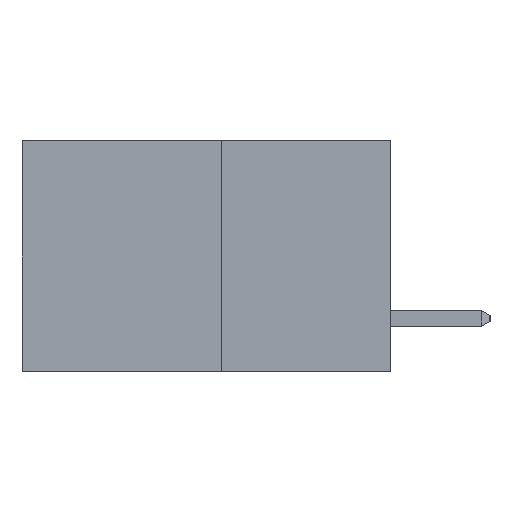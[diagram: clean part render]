
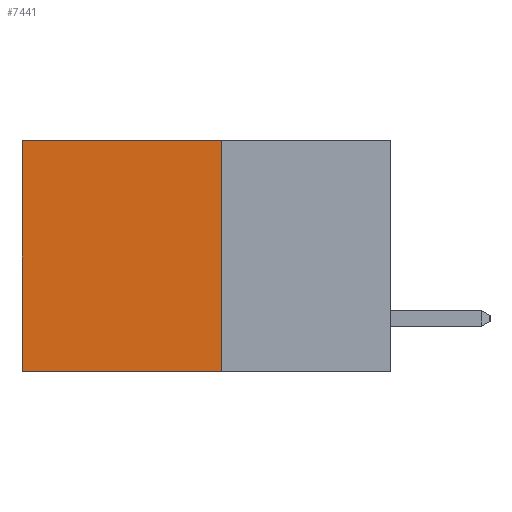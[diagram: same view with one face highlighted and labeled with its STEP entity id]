
A CAD part, left-side view. The second image highlights one B-rep face of the part: STEP entity #7441.
In plain terms, the highlighted planar face has unit normal (-1, 0, 0).
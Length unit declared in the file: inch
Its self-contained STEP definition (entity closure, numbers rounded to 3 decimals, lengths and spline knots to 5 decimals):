
#390 = CARTESIAN_POINT ( 'NONE',  ( 0.277, 0.27, -0.37 ) ) ;
#994 = ORIENTED_EDGE ( 'NONE', *, *, #7520, .T. ) ;
#1193 = CARTESIAN_POINT ( 'NONE',  ( 0.277, 0.27, -0.37 ) ) ;
#1425 = VERTEX_POINT ( 'NONE', #12397 ) ;
#1531 = DIRECTION ( 'NONE',  ( 0., 0., -1. ) ) ;
#1620 = LINE ( 'NONE', #11515, #12965 ) ;
#2081 = AXIS2_PLACEMENT_3D ( 'NONE', #390, #8205, #1531 ) ;
#2526 = CARTESIAN_POINT ( 'NONE',  ( 0.277, 0.27, 0. ) ) ;
#2541 = CARTESIAN_POINT ( 'NONE',  ( 0.277, 0.27, 0. ) ) ;
#3021 = VERTEX_POINT ( 'NONE', #4196 ) ;
#3161 = EDGE_LOOP ( 'NONE', ( #994, #9146, #4348, #8021 ) ) ;
#3484 = LINE ( 'NONE', #1193, #9038 ) ;
#3695 = LINE ( 'NONE', #11509, #6670 ) ;
#3814 = DIRECTION ( 'NONE',  ( 0., 0., -1. ) ) ;
#4196 = CARTESIAN_POINT ( 'NONE',  ( 0.277, 0.59, 0. ) ) ;
#4348 = ORIENTED_EDGE ( 'NONE', *, *, #13926, .F. ) ;
#6143 = LINE ( 'NONE', #2526, #10631 ) ;
#6670 = VECTOR ( 'NONE', #3814, 39.37008 ) ;
#6728 = VERTEX_POINT ( 'NONE', #13368 ) ;
#7095 = PLANE ( 'NONE',  #2081 ) ;
#7197 = DIRECTION ( 'NONE',  ( 0., 0., -1. ) ) ;
#7392 = EDGE_CURVE ( 'NONE', #8718, #3021, #6143, .T. ) ;
#7441 = ADVANCED_FACE ( 'NONE', ( #13134 ), #7095, .F. ) ;
#7520 = EDGE_CURVE ( 'NONE', #3021, #1425, #3695, .T. ) ;
#8021 = ORIENTED_EDGE ( 'NONE', *, *, #7392, .T. ) ;
#8205 = DIRECTION ( 'NONE',  ( 1., 0., 0. ) ) ;
#8608 = EDGE_CURVE ( 'NONE', #6728, #1425, #3484, .T. ) ;
#8718 = VERTEX_POINT ( 'NONE', #2541 ) ;
#9038 = VECTOR ( 'NONE', #11174, 39.37008 ) ;
#9146 = ORIENTED_EDGE ( 'NONE', *, *, #8608, .F. ) ;
#10631 = VECTOR ( 'NONE', #11392, 39.37008 ) ;
#11174 = DIRECTION ( 'NONE',  ( 0., 1., 0. ) ) ;
#11392 = DIRECTION ( 'NONE',  ( 0., 1., 0. ) ) ;
#11509 = CARTESIAN_POINT ( 'NONE',  ( 0.277, 0.59, -0.37 ) ) ;
#11515 = CARTESIAN_POINT ( 'NONE',  ( 0.277, 0.27, -0.37 ) ) ;
#12397 = CARTESIAN_POINT ( 'NONE',  ( 0.277, 0.59, -0.37 ) ) ;
#12965 = VECTOR ( 'NONE', #7197, 39.37008 ) ;
#13134 = FACE_OUTER_BOUND ( 'NONE', #3161, .T. ) ;
#13368 = CARTESIAN_POINT ( 'NONE',  ( 0.277, 0.27, -0.37 ) ) ;
#13926 = EDGE_CURVE ( 'NONE', #8718, #6728, #1620, .T. ) ;
